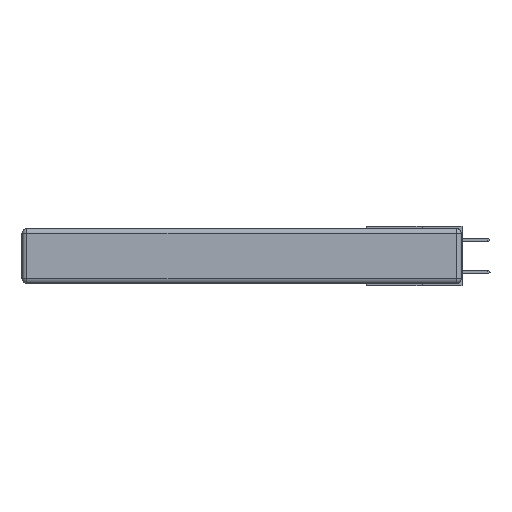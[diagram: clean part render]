
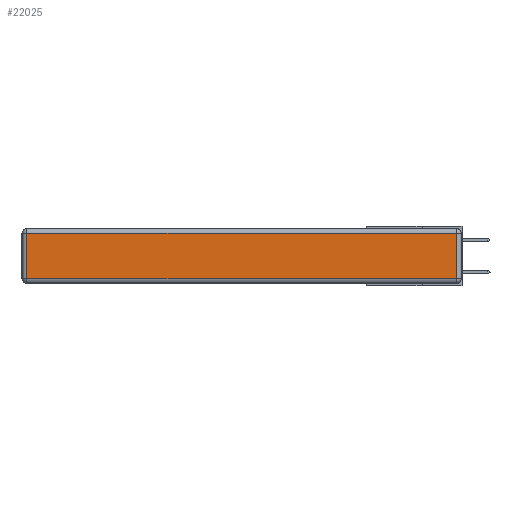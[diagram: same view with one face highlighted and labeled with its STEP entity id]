
A CAD part, left-side view. The second image highlights one B-rep face of the part: STEP entity #22025.
In plain terms, the highlighted planar face has unit normal (-1, 0, 0).
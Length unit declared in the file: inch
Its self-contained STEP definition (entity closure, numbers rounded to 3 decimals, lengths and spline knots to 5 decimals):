
#20 = VERTEX_POINT ( 'NONE', #568 ) ;
#29 = DIRECTION ( 'NONE',  ( 0., -1., 0. ) ) ;
#568 = CARTESIAN_POINT ( 'NONE',  ( 0., 0.03, -0.313 ) ) ;
#1646 = ORIENTED_EDGE ( 'NONE', *, *, #27798, .T. ) ;
#2529 = LINE ( 'NONE', #7789, #10815 ) ;
#2813 = CARTESIAN_POINT ( 'NONE',  ( 0., 2.72, -0.313 ) ) ;
#4581 = PLANE ( 'NONE',  #6207 ) ;
#4794 = EDGE_CURVE ( 'NONE', #10772, #32309, #17803, .T. ) ;
#5170 = VECTOR ( 'NONE', #13777, 39.37008 ) ;
#5651 = CARTESIAN_POINT ( 'NONE',  ( 0., 2.72, -0.343 ) ) ;
#5702 = EDGE_CURVE ( 'NONE', #20, #28015, #2529, .T. ) ;
#6207 = AXIS2_PLACEMENT_3D ( 'NONE', #24986, #7336, #22319 ) ;
#7336 = DIRECTION ( 'NONE',  ( -1., 0., 0. ) ) ;
#7505 = ORIENTED_EDGE ( 'NONE', *, *, #5702, .T. ) ;
#7789 = CARTESIAN_POINT ( 'NONE',  ( 0., 0.03, -0.343 ) ) ;
#8899 = CARTESIAN_POINT ( 'NONE',  ( 0., 2.72, -0.03 ) ) ;
#10240 = VECTOR ( 'NONE', #30085, 39.37008 ) ;
#10772 = VERTEX_POINT ( 'NONE', #8899 ) ;
#10815 = VECTOR ( 'NONE', #17061, 39.37008 ) ;
#12736 = VECTOR ( 'NONE', #29, 39.37008 ) ;
#13777 = DIRECTION ( 'NONE',  ( 0., 1., 0. ) ) ;
#14129 = CARTESIAN_POINT ( 'NONE',  ( 0., 0.03, -0.03 ) ) ;
#17061 = DIRECTION ( 'NONE',  ( 0., 0., 1. ) ) ;
#17615 = FACE_OUTER_BOUND ( 'NONE', #23496, .T. ) ;
#17803 = LINE ( 'NONE', #5651, #10240 ) ;
#20373 = CARTESIAN_POINT ( 'NONE',  ( 0., 2.75, -0.03 ) ) ;
#21894 = LINE ( 'NONE', #25361, #12736 ) ;
#22025 = ADVANCED_FACE ( 'NONE', ( #17615 ), #4581, .T. ) ;
#22319 = DIRECTION ( 'NONE',  ( 0., 0., 1. ) ) ;
#23055 = ORIENTED_EDGE ( 'NONE', *, *, #4794, .T. ) ;
#23462 = EDGE_CURVE ( 'NONE', #32309, #20, #21894, .T. ) ;
#23496 = EDGE_LOOP ( 'NONE', ( #25752, #7505, #1646, #23055 ) ) ;
#24986 = CARTESIAN_POINT ( 'NONE',  ( 0., 0., -0.343 ) ) ;
#25361 = CARTESIAN_POINT ( 'NONE',  ( 0., 0., -0.313 ) ) ;
#25752 = ORIENTED_EDGE ( 'NONE', *, *, #23462, .T. ) ;
#27433 = LINE ( 'NONE', #20373, #5170 ) ;
#27798 = EDGE_CURVE ( 'NONE', #28015, #10772, #27433, .T. ) ;
#28015 = VERTEX_POINT ( 'NONE', #14129 ) ;
#30085 = DIRECTION ( 'NONE',  ( 0., 0., -1. ) ) ;
#32309 = VERTEX_POINT ( 'NONE', #2813 ) ;
